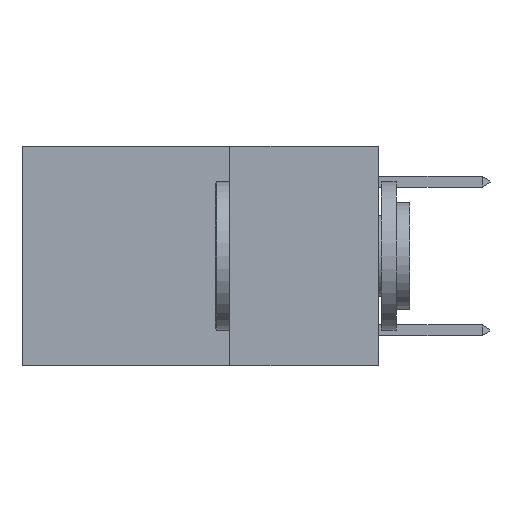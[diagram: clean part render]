
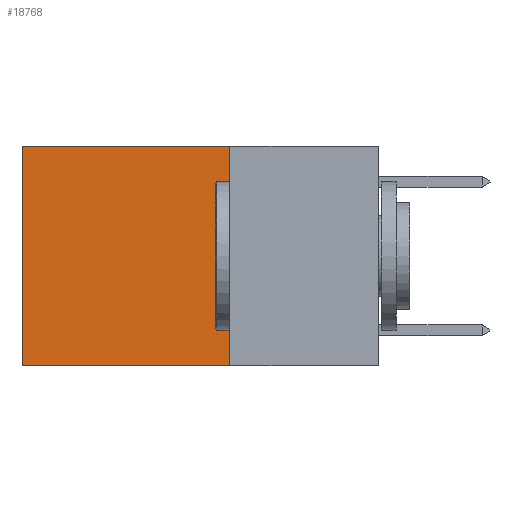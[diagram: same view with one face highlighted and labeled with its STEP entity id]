
A CAD part, left-side view. The second image highlights one B-rep face of the part: STEP entity #18768.
In plain terms, the highlighted planar face has unit normal (-1, 0, 0).
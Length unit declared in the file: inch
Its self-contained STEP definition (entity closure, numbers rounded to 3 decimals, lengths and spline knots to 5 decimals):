
#136 = VERTEX_POINT ( 'NONE', #17195 ) ;
#1093 = EDGE_CURVE ( 'NONE', #18841, #11725, #13419, .T. ) ;
#2324 = DIRECTION ( 'NONE',  ( 0., 1., 0. ) ) ;
#2756 = CARTESIAN_POINT ( 'NONE',  ( 0.2625, 0.25, 0. ) ) ;
#3125 = LINE ( 'NONE', #4510, #15582 ) ;
#4112 = DIRECTION ( 'NONE',  ( 1., 0., 0. ) ) ;
#4510 = CARTESIAN_POINT ( 'NONE',  ( 0.2625, 0.6, 0. ) ) ;
#4719 = EDGE_CURVE ( 'NONE', #11725, #136, #3125, .T. ) ;
#6121 = DIRECTION ( 'NONE',  ( 0., 0., -1. ) ) ;
#7458 = ORIENTED_EDGE ( 'NONE', *, *, #21012, .F. ) ;
#8022 = FACE_OUTER_BOUND ( 'NONE', #8717, .T. ) ;
#8717 = EDGE_LOOP ( 'NONE', ( #22709, #7458, #26484, #24289 ) ) ;
#10363 = CARTESIAN_POINT ( 'NONE',  ( 0.2625, 0.25, 0. ) ) ;
#10551 = LINE ( 'NONE', #25650, #11199 ) ;
#10558 = AXIS2_PLACEMENT_3D ( 'NONE', #10363, #4112, #6121 ) ;
#11199 = VECTOR ( 'NONE', #19069, 39.37008 ) ;
#11725 = VERTEX_POINT ( 'NONE', #16548 ) ;
#12027 = PLANE ( 'NONE',  #10558 ) ;
#13419 = LINE ( 'NONE', #14213, #19666 ) ;
#13832 = CARTESIAN_POINT ( 'NONE',  ( 0.2625, 0.25, -0.37 ) ) ;
#14213 = CARTESIAN_POINT ( 'NONE',  ( 0.2625, 0.25, 0. ) ) ;
#15582 = VECTOR ( 'NONE', #23326, 39.37008 ) ;
#16548 = CARTESIAN_POINT ( 'NONE',  ( 0.2625, 0.6, 0. ) ) ;
#17195 = CARTESIAN_POINT ( 'NONE',  ( 0.2625, 0.6, -0.37 ) ) ;
#18768 = ADVANCED_FACE ( 'NONE', ( #8022 ), #12027, .F. ) ;
#18841 = VERTEX_POINT ( 'NONE', #2756 ) ;
#19069 = DIRECTION ( 'NONE',  ( 0., 0., -1. ) ) ;
#19666 = VECTOR ( 'NONE', #2324, 39.37008 ) ;
#21012 = EDGE_CURVE ( 'NONE', #25878, #136, #24510, .T. ) ;
#22709 = ORIENTED_EDGE ( 'NONE', *, *, #4719, .T. ) ;
#23211 = VECTOR ( 'NONE', #26788, 39.37008 ) ;
#23326 = DIRECTION ( 'NONE',  ( 0., 0., -1. ) ) ;
#24289 = ORIENTED_EDGE ( 'NONE', *, *, #1093, .T. ) ;
#24510 = LINE ( 'NONE', #13832, #23211 ) ;
#25566 = EDGE_CURVE ( 'NONE', #18841, #25878, #10551, .T. ) ;
#25650 = CARTESIAN_POINT ( 'NONE',  ( 0.2625, 0.25, 0. ) ) ;
#25878 = VERTEX_POINT ( 'NONE', #26188 ) ;
#26188 = CARTESIAN_POINT ( 'NONE',  ( 0.2625, 0.25, -0.37 ) ) ;
#26484 = ORIENTED_EDGE ( 'NONE', *, *, #25566, .F. ) ;
#26788 = DIRECTION ( 'NONE',  ( 0., 1., 0. ) ) ;
